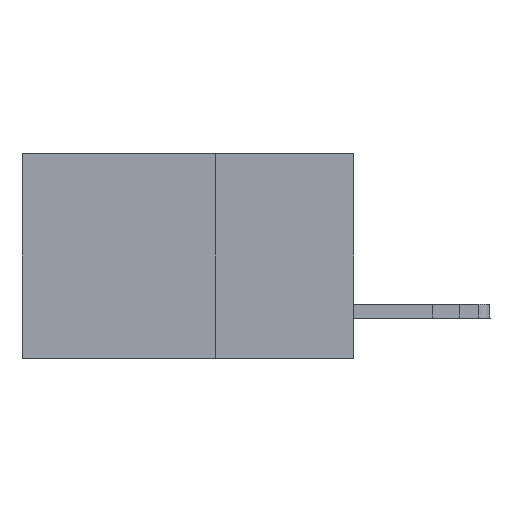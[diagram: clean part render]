
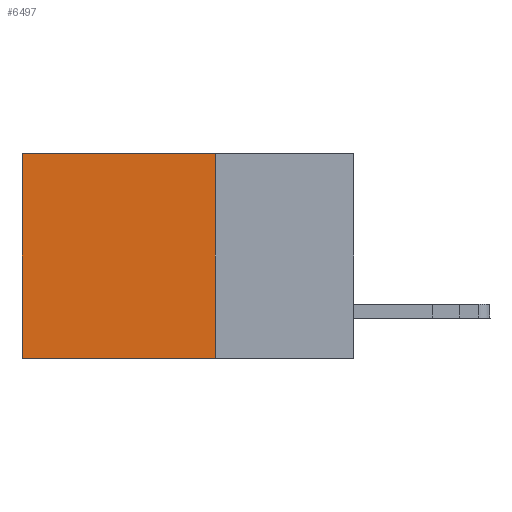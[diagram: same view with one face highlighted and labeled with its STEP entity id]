
A CAD part, left-side view. The second image highlights one B-rep face of the part: STEP entity #6497.
In plain terms, the highlighted planar face has unit normal (-1, 0, 0).
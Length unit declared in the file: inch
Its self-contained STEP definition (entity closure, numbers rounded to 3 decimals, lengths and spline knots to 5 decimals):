
#2028 = VECTOR ( 'NONE', #16092, 39.37008 ) ;
#2528 = CARTESIAN_POINT ( 'NONE',  ( 0.2875, 0.25, 0. ) ) ;
#2837 = CARTESIAN_POINT ( 'NONE',  ( 0.2875, 0.6, 0. ) ) ;
#3967 = VERTEX_POINT ( 'NONE', #8265 ) ;
#3997 = EDGE_CURVE ( 'NONE', #17791, #10495, #9667, .T. ) ;
#4145 = VERTEX_POINT ( 'NONE', #11626 ) ;
#4278 = CARTESIAN_POINT ( 'NONE',  ( 0.2875, 0.25, -0.37 ) ) ;
#4911 = EDGE_CURVE ( 'NONE', #3967, #4145, #15712, .T. ) ;
#5064 = FACE_OUTER_BOUND ( 'NONE', #5944, .T. ) ;
#5486 = EDGE_CURVE ( 'NONE', #17791, #3967, #8735, .T. ) ;
#5902 = CARTESIAN_POINT ( 'NONE',  ( 0.2875, 0.25, 0. ) ) ;
#5944 = EDGE_LOOP ( 'NONE', ( #15851, #18107, #11135, #8748 ) ) ;
#6284 = DIRECTION ( 'NONE',  ( 0., 1., 0. ) ) ;
#6497 = ADVANCED_FACE ( 'NONE', ( #5064 ), #18331, .F. ) ;
#7158 = DIRECTION ( 'NONE',  ( 0., 0., -1. ) ) ;
#7986 = EDGE_CURVE ( 'NONE', #10495, #4145, #11749, .T. ) ;
#8265 = CARTESIAN_POINT ( 'NONE',  ( 0.2875, 0.6, 0. ) ) ;
#8272 = DIRECTION ( 'NONE',  ( 0., 0., -1. ) ) ;
#8735 = LINE ( 'NONE', #5902, #14729 ) ;
#8748 = ORIENTED_EDGE ( 'NONE', *, *, #5486, .T. ) ;
#9201 = AXIS2_PLACEMENT_3D ( 'NONE', #2528, #9318, #8272 ) ;
#9318 = DIRECTION ( 'NONE',  ( 1., 0., 0. ) ) ;
#9667 = LINE ( 'NONE', #12573, #11589 ) ;
#10495 = VERTEX_POINT ( 'NONE', #4278 ) ;
#11135 = ORIENTED_EDGE ( 'NONE', *, *, #3997, .F. ) ;
#11589 = VECTOR ( 'NONE', #14353, 39.37008 ) ;
#11626 = CARTESIAN_POINT ( 'NONE',  ( 0.2875, 0.6, -0.37 ) ) ;
#11749 = LINE ( 'NONE', #17489, #2028 ) ;
#12573 = CARTESIAN_POINT ( 'NONE',  ( 0.2875, 0.25, 0. ) ) ;
#14353 = DIRECTION ( 'NONE',  ( 0., 0., -1. ) ) ;
#14729 = VECTOR ( 'NONE', #6284, 39.37008 ) ;
#15605 = VECTOR ( 'NONE', #7158, 39.37008 ) ;
#15712 = LINE ( 'NONE', #2837, #15605 ) ;
#15851 = ORIENTED_EDGE ( 'NONE', *, *, #4911, .T. ) ;
#16092 = DIRECTION ( 'NONE',  ( 0., 1., 0. ) ) ;
#17489 = CARTESIAN_POINT ( 'NONE',  ( 0.2875, 0.25, -0.37 ) ) ;
#17509 = CARTESIAN_POINT ( 'NONE',  ( 0.2875, 0.25, 0. ) ) ;
#17791 = VERTEX_POINT ( 'NONE', #17509 ) ;
#18107 = ORIENTED_EDGE ( 'NONE', *, *, #7986, .F. ) ;
#18331 = PLANE ( 'NONE',  #9201 ) ;
